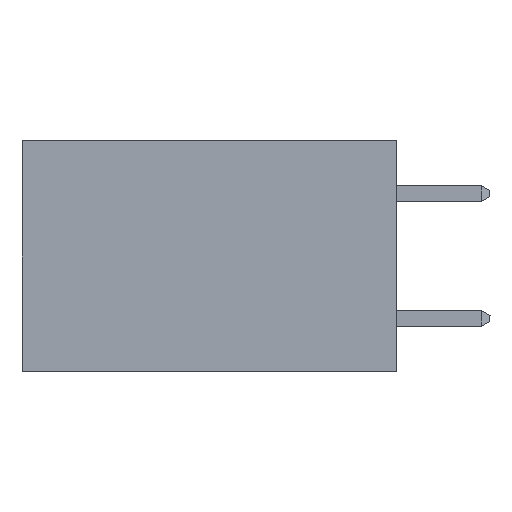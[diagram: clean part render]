
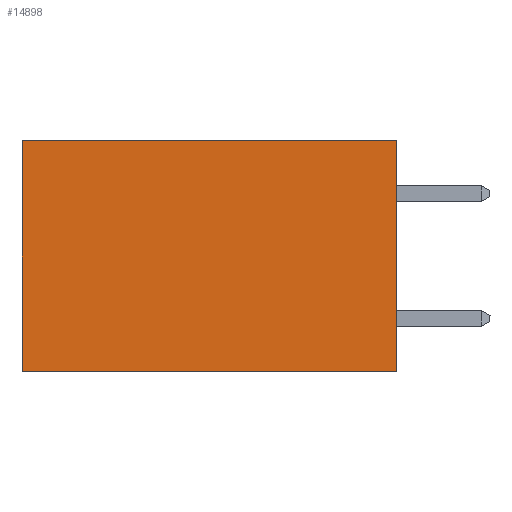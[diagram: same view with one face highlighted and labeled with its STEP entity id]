
A CAD part, left-side view. The second image highlights one B-rep face of the part: STEP entity #14898.
In plain terms, the highlighted planar face has unit normal (-1, 0, 0).
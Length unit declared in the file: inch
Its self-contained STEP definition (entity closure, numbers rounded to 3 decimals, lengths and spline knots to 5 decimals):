
#1420 = VERTEX_POINT ( 'NONE', #6948 ) ;
#2516 = ORIENTED_EDGE ( 'NONE', *, *, #7464, .F. ) ;
#2537 = VERTEX_POINT ( 'NONE', #11893 ) ;
#2675 = CARTESIAN_POINT ( 'NONE',  ( 0.2615, 0.6, -0.37 ) ) ;
#2676 = LINE ( 'NONE', #8744, #5508 ) ;
#3113 = EDGE_CURVE ( 'NONE', #14268, #3193, #3307, .T. ) ;
#3193 = VERTEX_POINT ( 'NONE', #2675 ) ;
#3307 = LINE ( 'NONE', #3483, #15100 ) ;
#3402 = DIRECTION ( 'NONE',  ( 0., 1., 0. ) ) ;
#3483 = CARTESIAN_POINT ( 'NONE',  ( 0.2615, 0., -0.37 ) ) ;
#3847 = AXIS2_PLACEMENT_3D ( 'NONE', #7479, #6298, #14533 ) ;
#4796 = VECTOR ( 'NONE', #15255, 39.37008 ) ;
#4825 = ORIENTED_EDGE ( 'NONE', *, *, #13449, .T. ) ;
#5091 = PLANE ( 'NONE',  #3847 ) ;
#5325 = FACE_OUTER_BOUND ( 'NONE', #10333, .T. ) ;
#5508 = VECTOR ( 'NONE', #8365, 39.37008 ) ;
#6298 = DIRECTION ( 'NONE',  ( 1., 0., 0. ) ) ;
#6948 = CARTESIAN_POINT ( 'NONE',  ( 0.2615, 0.6, 0. ) ) ;
#7464 = EDGE_CURVE ( 'NONE', #2537, #14268, #2676, .T. ) ;
#7479 = CARTESIAN_POINT ( 'NONE',  ( 0.2615, 0., -0.37 ) ) ;
#7999 = ORIENTED_EDGE ( 'NONE', *, *, #12697, .T. ) ;
#8330 = CARTESIAN_POINT ( 'NONE',  ( 0.2615, 0., 0. ) ) ;
#8365 = DIRECTION ( 'NONE',  ( 0., 0., -1. ) ) ;
#8744 = CARTESIAN_POINT ( 'NONE',  ( 0.2615, 0., -0.37 ) ) ;
#9561 = VECTOR ( 'NONE', #12791, 39.37008 ) ;
#10333 = EDGE_LOOP ( 'NONE', ( #7999, #13197, #2516, #4825 ) ) ;
#11182 = LINE ( 'NONE', #8330, #4796 ) ;
#11893 = CARTESIAN_POINT ( 'NONE',  ( 0.2615, 0., 0. ) ) ;
#12255 = LINE ( 'NONE', #12866, #9561 ) ;
#12697 = EDGE_CURVE ( 'NONE', #1420, #3193, #12255, .T. ) ;
#12791 = DIRECTION ( 'NONE',  ( 0., 0., -1. ) ) ;
#12866 = CARTESIAN_POINT ( 'NONE',  ( 0.2615, 0.6, -0.37 ) ) ;
#13197 = ORIENTED_EDGE ( 'NONE', *, *, #3113, .F. ) ;
#13449 = EDGE_CURVE ( 'NONE', #2537, #1420, #11182, .T. ) ;
#14268 = VERTEX_POINT ( 'NONE', #15471 ) ;
#14533 = DIRECTION ( 'NONE',  ( 0., 0., -1. ) ) ;
#14898 = ADVANCED_FACE ( 'NONE', ( #5325 ), #5091, .F. ) ;
#15100 = VECTOR ( 'NONE', #3402, 39.37008 ) ;
#15255 = DIRECTION ( 'NONE',  ( 0., 1., 0. ) ) ;
#15471 = CARTESIAN_POINT ( 'NONE',  ( 0.2615, 0., -0.37 ) ) ;
